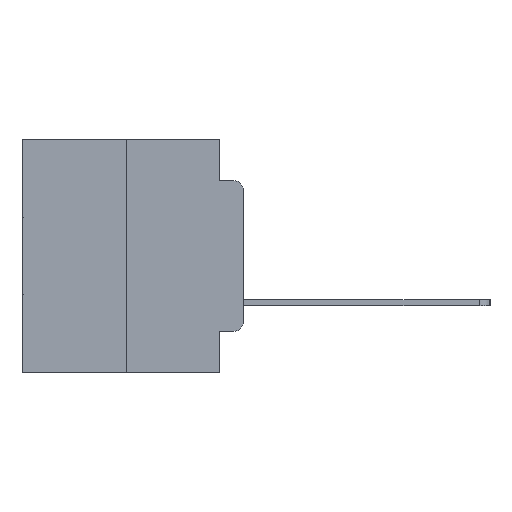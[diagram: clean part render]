
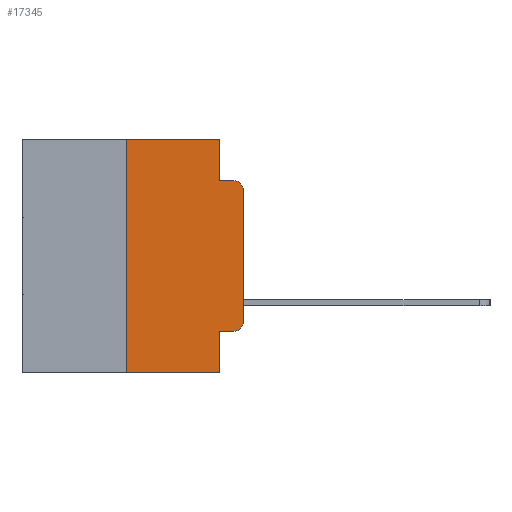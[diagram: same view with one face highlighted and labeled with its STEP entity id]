
A CAD part, left-side view. The second image highlights one B-rep face of the part: STEP entity #17345.
In plain terms, the highlighted planar face has unit normal (-1, 0, 0).
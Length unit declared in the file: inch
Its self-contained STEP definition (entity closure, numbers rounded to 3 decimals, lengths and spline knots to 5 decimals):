
#451 = AXIS2_PLACEMENT_3D ( 'NONE', #4706, #26922, #13697 ) ;
#504 = CARTESIAN_POINT ( 'NONE',  ( 0., 0.051, -0.4115 ) ) ;
#713 = CIRCLE ( 'NONE', #9906, 0.02 ) ;
#848 = EDGE_LOOP ( 'NONE', ( #8373, #13171, #4375, #4976, #2737, #26318, #8599, #7679, #4036, #22430 ) ) ;
#2071 = CARTESIAN_POINT ( 'NONE',  ( 0., 0.25, 0. ) ) ;
#2480 = LINE ( 'NONE', #15658, #13706 ) ;
#2737 = ORIENTED_EDGE ( 'NONE', *, *, #16080, .F. ) ;
#3667 = LINE ( 'NONE', #5055, #25926 ) ;
#3934 = VERTEX_POINT ( 'NONE', #25497 ) ;
#4036 = ORIENTED_EDGE ( 'NONE', *, *, #7453, .T. ) ;
#4065 = CARTESIAN_POINT ( 'NONE',  ( 0., 0.051, 0. ) ) ;
#4302 = VERTEX_POINT ( 'NONE', #6761 ) ;
#4375 = ORIENTED_EDGE ( 'NONE', *, *, #17920, .F. ) ;
#4706 = CARTESIAN_POINT ( 'NONE',  ( 0., 0.473, 0. ) ) ;
#4976 = ORIENTED_EDGE ( 'NONE', *, *, #14915, .F. ) ;
#5055 = CARTESIAN_POINT ( 'NONE',  ( 0., 0.473, -0.5 ) ) ;
#5570 = CARTESIAN_POINT ( 'NONE',  ( 0., 0.02, -0.4115 ) ) ;
#5907 = DIRECTION ( 'NONE',  ( -1., 0., 0. ) ) ;
#5958 = EDGE_CURVE ( 'NONE', #15772, #4302, #713, .T. ) ;
#5969 = LINE ( 'NONE', #8874, #23011 ) ;
#6205 = VECTOR ( 'NONE', #26722, 39.37008 ) ;
#6485 = CARTESIAN_POINT ( 'NONE',  ( 0., 0.02, -0.3915 ) ) ;
#6761 = CARTESIAN_POINT ( 'NONE',  ( 0., 0., -0.3915 ) ) ;
#7129 = VECTOR ( 'NONE', #15518, 39.37008 ) ;
#7296 = DIRECTION ( 'NONE',  ( 0., -1., 0. ) ) ;
#7453 = EDGE_CURVE ( 'NONE', #8461, #15772, #13658, .T. ) ;
#7679 = ORIENTED_EDGE ( 'NONE', *, *, #8949, .F. ) ;
#7684 = VECTOR ( 'NONE', #19680, 39.37008 ) ;
#7856 = VERTEX_POINT ( 'NONE', #20304 ) ;
#8373 = ORIENTED_EDGE ( 'NONE', *, *, #23814, .T. ) ;
#8461 = VERTEX_POINT ( 'NONE', #9193 ) ;
#8597 = CARTESIAN_POINT ( 'NONE',  ( 0., 0.25, 0. ) ) ;
#8599 = ORIENTED_EDGE ( 'NONE', *, *, #27125, .T. ) ;
#8726 = DIRECTION ( 'NONE',  ( 0., 0., -1. ) ) ;
#8874 = CARTESIAN_POINT ( 'NONE',  ( 0., 0.473, 0. ) ) ;
#8949 = EDGE_CURVE ( 'NONE', #8461, #22300, #19539, .T. ) ;
#9048 = DIRECTION ( 'NONE',  ( 0., 0., 1. ) ) ;
#9193 = CARTESIAN_POINT ( 'NONE',  ( 0., 0.051, -0.4115 ) ) ;
#9689 = VECTOR ( 'NONE', #9048, 39.37008 ) ;
#9906 = AXIS2_PLACEMENT_3D ( 'NONE', #6485, #22039, #8726 ) ;
#11090 = DIRECTION ( 'NONE',  ( 0., -1., 0. ) ) ;
#11545 = AXIS2_PLACEMENT_3D ( 'NONE', #19252, #5907, #21481 ) ;
#11760 = DIRECTION ( 'NONE',  ( 0., -1., 0. ) ) ;
#12682 = VERTEX_POINT ( 'NONE', #26252 ) ;
#13058 = LINE ( 'NONE', #2071, #7129 ) ;
#13171 = ORIENTED_EDGE ( 'NONE', *, *, #22358, .T. ) ;
#13197 = FACE_OUTER_BOUND ( 'NONE', #848, .T. ) ;
#13427 = EDGE_CURVE ( 'NONE', #25096, #18424, #13058, .T. ) ;
#13658 = LINE ( 'NONE', #504, #24730 ) ;
#13697 = DIRECTION ( 'NONE',  ( 0., 0., -1. ) ) ;
#13706 = VECTOR ( 'NONE', #17899, 39.37008 ) ;
#14592 = CARTESIAN_POINT ( 'NONE',  ( 0., 0.051, -0.5 ) ) ;
#14915 = EDGE_CURVE ( 'NONE', #12682, #7856, #2480, .T. ) ;
#15518 = DIRECTION ( 'NONE',  ( 0., 0., 1. ) ) ;
#15641 = LINE ( 'NONE', #24549, #9689 ) ;
#15658 = CARTESIAN_POINT ( 'NONE',  ( 0., 0.051, 0. ) ) ;
#15772 = VERTEX_POINT ( 'NONE', #5570 ) ;
#16080 = EDGE_CURVE ( 'NONE', #18424, #12682, #5969, .T. ) ;
#17345 = ADVANCED_FACE ( 'NONE', ( #13197 ), #24717, .F. ) ;
#17774 = CARTESIAN_POINT ( 'NONE',  ( 0., 0.25, -0.5 ) ) ;
#17899 = DIRECTION ( 'NONE',  ( 0., 0., -1. ) ) ;
#17920 = EDGE_CURVE ( 'NONE', #7856, #26826, #27335, .T. ) ;
#18424 = VERTEX_POINT ( 'NONE', #8597 ) ;
#19252 = CARTESIAN_POINT ( 'NONE',  ( 0., 0.02, -0.1085 ) ) ;
#19539 = LINE ( 'NONE', #4065, #7684 ) ;
#19600 = CARTESIAN_POINT ( 'NONE',  ( 0., 0.02, -0.0885 ) ) ;
#19680 = DIRECTION ( 'NONE',  ( 0., 0., -1. ) ) ;
#20304 = CARTESIAN_POINT ( 'NONE',  ( 0., 0.051, -0.0885 ) ) ;
#21481 = DIRECTION ( 'NONE',  ( 0., 0., -1. ) ) ;
#22039 = DIRECTION ( 'NONE',  ( -1., 0., 0. ) ) ;
#22300 = VERTEX_POINT ( 'NONE', #14592 ) ;
#22358 = EDGE_CURVE ( 'NONE', #3934, #26826, #25346, .T. ) ;
#22430 = ORIENTED_EDGE ( 'NONE', *, *, #5958, .T. ) ;
#23011 = VECTOR ( 'NONE', #11090, 39.37008 ) ;
#23814 = EDGE_CURVE ( 'NONE', #4302, #3934, #15641, .T. ) ;
#24549 = CARTESIAN_POINT ( 'NONE',  ( 0., 0., 0. ) ) ;
#24717 = PLANE ( 'NONE',  #451 ) ;
#24730 = VECTOR ( 'NONE', #11760, 39.37008 ) ;
#25096 = VERTEX_POINT ( 'NONE', #17774 ) ;
#25346 = CIRCLE ( 'NONE', #11545, 0.02 ) ;
#25497 = CARTESIAN_POINT ( 'NONE',  ( 0., 0., -0.1085 ) ) ;
#25926 = VECTOR ( 'NONE', #7296, 39.37008 ) ;
#26252 = CARTESIAN_POINT ( 'NONE',  ( 0., 0.051, 0. ) ) ;
#26318 = ORIENTED_EDGE ( 'NONE', *, *, #13427, .F. ) ;
#26626 = CARTESIAN_POINT ( 'NONE',  ( 0., 0.051, -0.0885 ) ) ;
#26722 = DIRECTION ( 'NONE',  ( 0., -1., 0. ) ) ;
#26826 = VERTEX_POINT ( 'NONE', #19600 ) ;
#26922 = DIRECTION ( 'NONE',  ( 1., 0., 0. ) ) ;
#27125 = EDGE_CURVE ( 'NONE', #25096, #22300, #3667, .T. ) ;
#27335 = LINE ( 'NONE', #26626, #6205 ) ;
